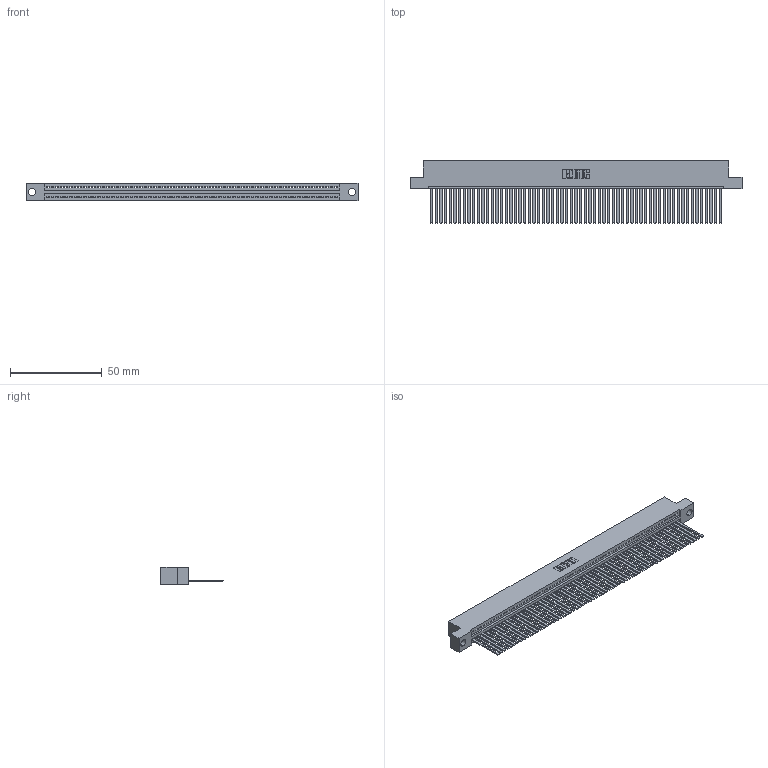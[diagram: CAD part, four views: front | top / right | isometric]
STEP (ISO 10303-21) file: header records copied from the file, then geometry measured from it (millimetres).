
FILE_DESCRIPTION (( 'STEP AP203' ), '1' );
FILE_NAME ('345-063-544-104.STEP', '2019-10-11T11:57:11', ( '' ), ( '' ), 'SwSTEP 2.0', 'SolidWorks 2016', '' );
FILE_SCHEMA (( 'CONFIG_CONTROL_DESIGN' ));
Length unit declared in the file: inch
Products named in the file (3): 345-063-544-104; 345 Part_Flush Mounting Lugs - 0.156 Dia-TH; 345-292-001_345-293-144
Assembly tree (64 placements, depth 2):
  345-063-544-104
    345 Part_Flush Mounting Lugs - 0.156 Dia-TH
    345-292-001_345-293-144  x63
Bounding box: 181.23 x 33.96 x 9.4 mm (x, y, z)
Volume: 18027.1 mm3; surface area: 26241 mm2
Topology: 64 solids, 64 shells, 3402 faces, 10295 edges, 6778 vertices
Faces by surface type: plane 2348, cylinder 1054
Entity records: 44407 total; most frequent: CARTESIAN_POINT 7697, ORIENTED_EDGE 7694, DIRECTION 6689, EDGE_CURVE 3847, LINE 3467, VECTOR 3467, VERTEX_POINT 2562, AXIS2_PLACEMENT_3D 1611
